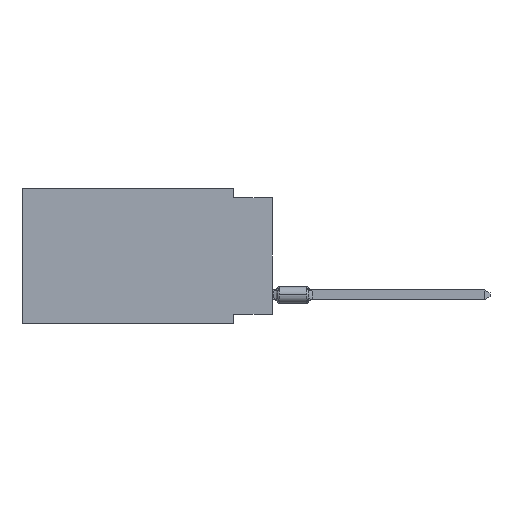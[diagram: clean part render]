
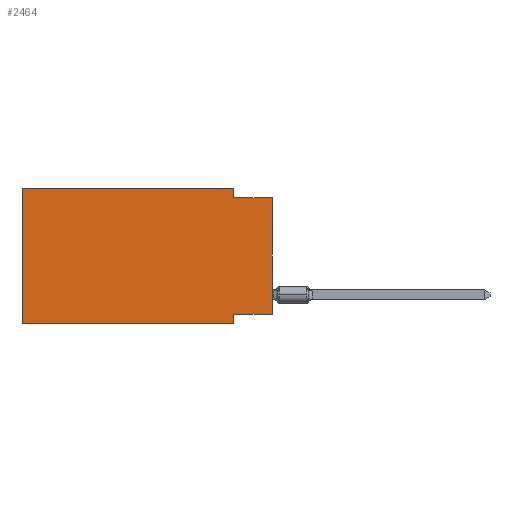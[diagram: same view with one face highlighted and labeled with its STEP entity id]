
A CAD part, left-side view. The second image highlights one B-rep face of the part: STEP entity #2464.
In plain terms, the highlighted planar face has unit normal (-1, 0, 0).
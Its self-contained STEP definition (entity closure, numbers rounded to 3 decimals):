
#316 = DIRECTION ( 'NONE',  ( 0., -1., 0. ) ) ;
#506 = EDGE_CURVE ( 'NONE', #14472, #7603, #1555, .T. ) ;
#638 = EDGE_CURVE ( 'NONE', #7519, #8892, #6238, .T. ) ;
#823 = VECTOR ( 'NONE', #316, 1000. ) ;
#1014 = LINE ( 'NONE', #7299, #3807 ) ;
#1164 = VERTEX_POINT ( 'NONE', #1729 ) ;
#1555 = LINE ( 'NONE', #10599, #2323 ) ;
#1729 = CARTESIAN_POINT ( 'NONE',  ( 0., 16.383, -8.89 ) ) ;
#1750 = PLANE ( 'NONE',  #6560 ) ;
#2030 = EDGE_CURVE ( 'NONE', #7587, #11776, #13162, .T. ) ;
#2201 = EDGE_CURVE ( 'NONE', #1164, #5460, #5179, .T. ) ;
#2323 = VECTOR ( 'NONE', #3059, 1000. ) ;
#2464 = ADVANCED_FACE ( 'NONE', ( #13138 ), #1750, .F. ) ;
#2592 = CARTESIAN_POINT ( 'NONE',  ( 0., 16.383, 0. ) ) ;
#3059 = DIRECTION ( 'NONE',  ( 0., 0., -1. ) ) ;
#3807 = VECTOR ( 'NONE', #12327, 1000. ) ;
#3842 = DIRECTION ( 'NONE',  ( 0., 0., 1. ) ) ;
#4083 = ORIENTED_EDGE ( 'NONE', *, *, #506, .F. ) ;
#4100 = CARTESIAN_POINT ( 'NONE',  ( 0., 16.383, -8.89 ) ) ;
#4709 = ORIENTED_EDGE ( 'NONE', *, *, #8391, .T. ) ;
#5179 = LINE ( 'NONE', #2592, #8707 ) ;
#5398 = EDGE_CURVE ( 'NONE', #7519, #14472, #1014, .T. ) ;
#5460 = VERTEX_POINT ( 'NONE', #7618 ) ;
#5595 = DIRECTION ( 'NONE',  ( 1., 0., 0. ) ) ;
#6238 = LINE ( 'NONE', #8914, #9002 ) ;
#6560 = AXIS2_PLACEMENT_3D ( 'NONE', #11964, #5595, #15395 ) ;
#7004 = CARTESIAN_POINT ( 'NONE',  ( 0., 2.54, -0.635 ) ) ;
#7299 = CARTESIAN_POINT ( 'NONE',  ( 0., 0., -8.255 ) ) ;
#7365 = ORIENTED_EDGE ( 'NONE', *, *, #5398, .F. ) ;
#7519 = VERTEX_POINT ( 'NONE', #10594 ) ;
#7587 = VERTEX_POINT ( 'NONE', #13027 ) ;
#7603 = VERTEX_POINT ( 'NONE', #10422 ) ;
#7618 = CARTESIAN_POINT ( 'NONE',  ( 0., 16.383, 0. ) ) ;
#8236 = CARTESIAN_POINT ( 'NONE',  ( 0., 0., -0.635 ) ) ;
#8391 = EDGE_CURVE ( 'NONE', #1164, #7603, #15577, .T. ) ;
#8707 = VECTOR ( 'NONE', #3842, 1000. ) ;
#8892 = VERTEX_POINT ( 'NONE', #11005 ) ;
#8914 = CARTESIAN_POINT ( 'NONE',  ( 0., 0., 0. ) ) ;
#9002 = VECTOR ( 'NONE', #11515, 1000. ) ;
#9479 = LINE ( 'NONE', #8236, #11498 ) ;
#10422 = CARTESIAN_POINT ( 'NONE',  ( 0., 2.54, -8.89 ) ) ;
#10566 = ORIENTED_EDGE ( 'NONE', *, *, #12298, .F. ) ;
#10594 = CARTESIAN_POINT ( 'NONE',  ( 0., 0., -8.255 ) ) ;
#10599 = CARTESIAN_POINT ( 'NONE',  ( 0., 2.54, -8.89 ) ) ;
#11005 = CARTESIAN_POINT ( 'NONE',  ( 0., 0., -0.635 ) ) ;
#11341 = ORIENTED_EDGE ( 'NONE', *, *, #638, .T. ) ;
#11420 = VECTOR ( 'NONE', #15742, 1000. ) ;
#11498 = VECTOR ( 'NONE', #12080, 1000. ) ;
#11515 = DIRECTION ( 'NONE',  ( 0., 0., 1. ) ) ;
#11776 = VERTEX_POINT ( 'NONE', #7004 ) ;
#11964 = CARTESIAN_POINT ( 'NONE',  ( 0., 16.383, 0. ) ) ;
#12077 = ORIENTED_EDGE ( 'NONE', *, *, #15208, .F. ) ;
#12080 = DIRECTION ( 'NONE',  ( 0., -1., 0. ) ) ;
#12298 = EDGE_CURVE ( 'NONE', #5460, #7587, #13134, .T. ) ;
#12327 = DIRECTION ( 'NONE',  ( 0., 1., 0. ) ) ;
#12733 = EDGE_LOOP ( 'NONE', ( #11341, #12077, #15250, #10566, #15337, #4709, #4083, #7365 ) ) ;
#13027 = CARTESIAN_POINT ( 'NONE',  ( 0., 2.54, 0. ) ) ;
#13134 = LINE ( 'NONE', #15391, #823 ) ;
#13138 = FACE_OUTER_BOUND ( 'NONE', #12733, .T. ) ;
#13162 = LINE ( 'NONE', #13490, #13760 ) ;
#13490 = CARTESIAN_POINT ( 'NONE',  ( 0., 2.54, 0. ) ) ;
#13760 = VECTOR ( 'NONE', #14983, 1000. ) ;
#14013 = CARTESIAN_POINT ( 'NONE',  ( 0., 2.54, -8.255 ) ) ;
#14472 = VERTEX_POINT ( 'NONE', #14013 ) ;
#14983 = DIRECTION ( 'NONE',  ( 0., 0., -1. ) ) ;
#15208 = EDGE_CURVE ( 'NONE', #11776, #8892, #9479, .T. ) ;
#15250 = ORIENTED_EDGE ( 'NONE', *, *, #2030, .F. ) ;
#15337 = ORIENTED_EDGE ( 'NONE', *, *, #2201, .F. ) ;
#15391 = CARTESIAN_POINT ( 'NONE',  ( 0., 16.383, 0. ) ) ;
#15395 = DIRECTION ( 'NONE',  ( 0., 0., -1. ) ) ;
#15577 = LINE ( 'NONE', #4100, #11420 ) ;
#15742 = DIRECTION ( 'NONE',  ( 0., -1., 0. ) ) ;
